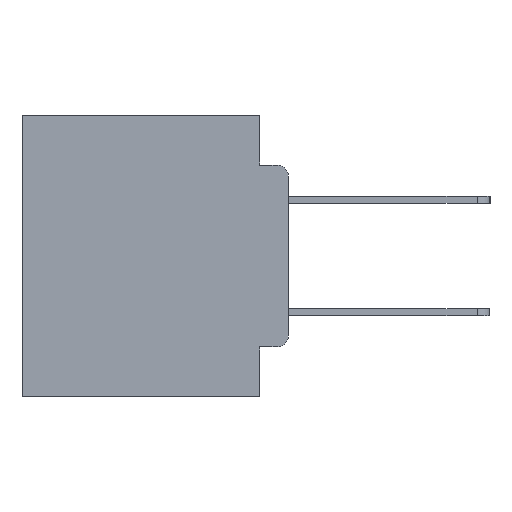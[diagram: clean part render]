
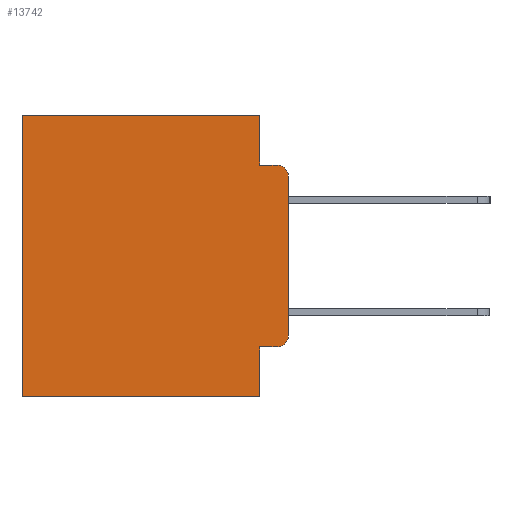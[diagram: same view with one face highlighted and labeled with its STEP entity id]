
A CAD part, left-side view. The second image highlights one B-rep face of the part: STEP entity #13742.
In plain terms, the highlighted planar face has unit normal (-1, 0, 0).
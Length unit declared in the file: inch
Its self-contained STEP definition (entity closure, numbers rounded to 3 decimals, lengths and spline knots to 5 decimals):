
#334 = ORIENTED_EDGE ( 'NONE', *, *, #27872, .T. ) ;
#545 = EDGE_CURVE ( 'NONE', #24810, #17333, #1311, .T. ) ;
#672 = CARTESIAN_POINT ( 'NONE',  ( 0.298, 0.02, -0.0885 ) ) ;
#682 = CARTESIAN_POINT ( 'NONE',  ( 0.298, 0.473, 0. ) ) ;
#844 = EDGE_CURVE ( 'NONE', #1964, #20528, #11742, .T. ) ;
#1087 = VERTEX_POINT ( 'NONE', #6576 ) ;
#1311 = LINE ( 'NONE', #11353, #24800 ) ;
#1792 = DIRECTION ( 'NONE',  ( -1., 0., 0. ) ) ;
#1964 = VERTEX_POINT ( 'NONE', #5483 ) ;
#2164 = LINE ( 'NONE', #6914, #13666 ) ;
#2759 = DIRECTION ( 'NONE',  ( -1., 0., 0. ) ) ;
#2830 = ORIENTED_EDGE ( 'NONE', *, *, #8960, .T. ) ;
#3038 = DIRECTION ( 'NONE',  ( 0., 0., -1. ) ) ;
#3194 = FACE_OUTER_BOUND ( 'NONE', #25303, .T. ) ;
#4149 = CARTESIAN_POINT ( 'NONE',  ( 0.298, 0., -0.5 ) ) ;
#4902 = VERTEX_POINT ( 'NONE', #672 ) ;
#5464 = AXIS2_PLACEMENT_3D ( 'NONE', #8690, #24480, #10965 ) ;
#5471 = ORIENTED_EDGE ( 'NONE', *, *, #844, .F. ) ;
#5483 = CARTESIAN_POINT ( 'NONE',  ( 0.298, 0., -0.1085 ) ) ;
#5666 = EDGE_CURVE ( 'NONE', #15530, #1087, #10749, .T. ) ;
#5973 = CIRCLE ( 'NONE', #22681, 0.02 ) ;
#6118 = ORIENTED_EDGE ( 'NONE', *, *, #11179, .T. ) ;
#6370 = PLANE ( 'NONE',  #5464 ) ;
#6507 = LINE ( 'NONE', #19722, #24577 ) ;
#6576 = CARTESIAN_POINT ( 'NONE',  ( 0.298, 0.473, -0.5 ) ) ;
#6914 = CARTESIAN_POINT ( 'NONE',  ( 0.298, 0.051, 0. ) ) ;
#7800 = VECTOR ( 'NONE', #3038, 39.37008 ) ;
#8256 = DIRECTION ( 'NONE',  ( 0., 1., 0. ) ) ;
#8438 = DIRECTION ( 'NONE',  ( 0., 0., -1. ) ) ;
#8690 = CARTESIAN_POINT ( 'NONE',  ( 0.298, 0., 0. ) ) ;
#8858 = VECTOR ( 'NONE', #8256, 39.37008 ) ;
#8960 = EDGE_CURVE ( 'NONE', #23540, #20742, #20168, .T. ) ;
#9216 = DIRECTION ( 'NONE',  ( 0., -1., 0. ) ) ;
#9330 = CARTESIAN_POINT ( 'NONE',  ( 0.298, 0., 0. ) ) ;
#10137 = ORIENTED_EDGE ( 'NONE', *, *, #22523, .F. ) ;
#10641 = CARTESIAN_POINT ( 'NONE',  ( 0.298, 0.051, -0.0885 ) ) ;
#10749 = LINE ( 'NONE', #4149, #28008 ) ;
#10965 = DIRECTION ( 'NONE',  ( 0., 0., -1. ) ) ;
#11109 = CARTESIAN_POINT ( 'NONE',  ( 0.298, 0.051, -0.0885 ) ) ;
#11179 = EDGE_CURVE ( 'NONE', #17333, #20528, #24264, .T. ) ;
#11353 = CARTESIAN_POINT ( 'NONE',  ( 0.298, 0.051, -0.4115 ) ) ;
#11742 = LINE ( 'NONE', #9330, #21615 ) ;
#12686 = EDGE_CURVE ( 'NONE', #23540, #20265, #2164, .T. ) ;
#13048 = DIRECTION ( 'NONE',  ( 0., -1., 0. ) ) ;
#13666 = VECTOR ( 'NONE', #20996, 39.37008 ) ;
#13708 = CARTESIAN_POINT ( 'NONE',  ( 0.298, 0.473, 0. ) ) ;
#13742 = ADVANCED_FACE ( 'NONE', ( #3194 ), #6370, .F. ) ;
#14491 = CARTESIAN_POINT ( 'NONE',  ( 0.298, 0.051, 0. ) ) ;
#14816 = CARTESIAN_POINT ( 'NONE',  ( 0.298, 0.051, -0.4115 ) ) ;
#15510 = CARTESIAN_POINT ( 'NONE',  ( 0.298, 0.02, -0.1085 ) ) ;
#15530 = VERTEX_POINT ( 'NONE', #16221 ) ;
#16104 = AXIS2_PLACEMENT_3D ( 'NONE', #16443, #2759, #18719 ) ;
#16221 = CARTESIAN_POINT ( 'NONE',  ( 0.298, 0.051, -0.5 ) ) ;
#16443 = CARTESIAN_POINT ( 'NONE',  ( 0.298, 0.02, -0.3915 ) ) ;
#17129 = ORIENTED_EDGE ( 'NONE', *, *, #545, .T. ) ;
#17333 = VERTEX_POINT ( 'NONE', #20769 ) ;
#17790 = DIRECTION ( 'NONE',  ( 0., 0., -1. ) ) ;
#18719 = DIRECTION ( 'NONE',  ( 0., 0., -1. ) ) ;
#18965 = ORIENTED_EDGE ( 'NONE', *, *, #24927, .F. ) ;
#19130 = ORIENTED_EDGE ( 'NONE', *, *, #5666, .F. ) ;
#19722 = CARTESIAN_POINT ( 'NONE',  ( 0.298, 0.051, 0. ) ) ;
#19729 = CARTESIAN_POINT ( 'NONE',  ( 0.298, 0., -0.3915 ) ) ;
#20168 = LINE ( 'NONE', #26303, #8858 ) ;
#20265 = VERTEX_POINT ( 'NONE', #11109 ) ;
#20528 = VERTEX_POINT ( 'NONE', #19729 ) ;
#20742 = VERTEX_POINT ( 'NONE', #13708 ) ;
#20769 = CARTESIAN_POINT ( 'NONE',  ( 0.298, 0.02, -0.4115 ) ) ;
#20913 = LINE ( 'NONE', #10641, #26169 ) ;
#20996 = DIRECTION ( 'NONE',  ( 0., 0., -1. ) ) ;
#21615 = VECTOR ( 'NONE', #28688, 39.37008 ) ;
#22523 = EDGE_CURVE ( 'NONE', #24810, #15530, #6507, .T. ) ;
#22681 = AXIS2_PLACEMENT_3D ( 'NONE', #15510, #1792, #17790 ) ;
#22802 = ORIENTED_EDGE ( 'NONE', *, *, #27578, .T. ) ;
#23540 = VERTEX_POINT ( 'NONE', #14491 ) ;
#24264 = CIRCLE ( 'NONE', #16104, 0.02 ) ;
#24466 = DIRECTION ( 'NONE',  ( 0., 1., 0. ) ) ;
#24480 = DIRECTION ( 'NONE',  ( 1., 0., 0. ) ) ;
#24577 = VECTOR ( 'NONE', #8438, 39.37008 ) ;
#24709 = ORIENTED_EDGE ( 'NONE', *, *, #12686, .F. ) ;
#24800 = VECTOR ( 'NONE', #9216, 39.37008 ) ;
#24810 = VERTEX_POINT ( 'NONE', #14816 ) ;
#24927 = EDGE_CURVE ( 'NONE', #20265, #4902, #20913, .T. ) ;
#25115 = LINE ( 'NONE', #682, #7800 ) ;
#25303 = EDGE_LOOP ( 'NONE', ( #5471, #334, #18965, #24709, #2830, #22802, #19130, #10137, #17129, #6118 ) ) ;
#26169 = VECTOR ( 'NONE', #13048, 39.37008 ) ;
#26303 = CARTESIAN_POINT ( 'NONE',  ( 0.298, 0., 0. ) ) ;
#27578 = EDGE_CURVE ( 'NONE', #20742, #1087, #25115, .T. ) ;
#27872 = EDGE_CURVE ( 'NONE', #1964, #4902, #5973, .T. ) ;
#28008 = VECTOR ( 'NONE', #24466, 39.37008 ) ;
#28688 = DIRECTION ( 'NONE',  ( 0., 0., -1. ) ) ;
